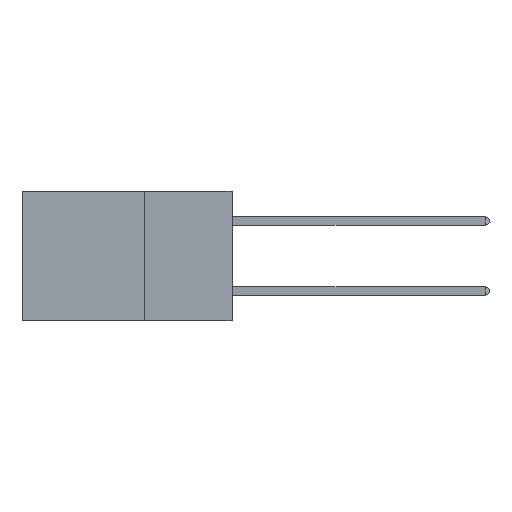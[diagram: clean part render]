
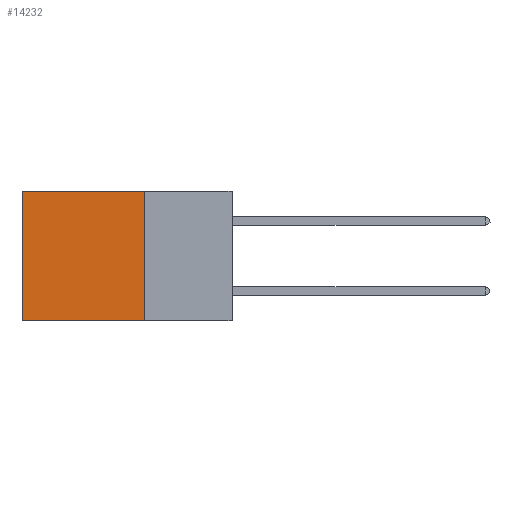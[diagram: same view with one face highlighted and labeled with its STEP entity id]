
A CAD part, left-side view. The second image highlights one B-rep face of the part: STEP entity #14232.
In plain terms, the highlighted planar face has unit normal (-1, 0, 0).
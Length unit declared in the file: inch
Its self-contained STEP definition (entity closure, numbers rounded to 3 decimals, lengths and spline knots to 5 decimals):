
#116 = DIRECTION ( 'NONE',  ( 0., 1., 0. ) ) ;
#477 = VERTEX_POINT ( 'NONE', #4011 ) ;
#758 = CARTESIAN_POINT ( 'NONE',  ( 0.2875, 0.25, 0. ) ) ;
#1013 = CARTESIAN_POINT ( 'NONE',  ( 0.2875, 0.25, -0.37 ) ) ;
#1071 = VERTEX_POINT ( 'NONE', #6090 ) ;
#1151 = ORIENTED_EDGE ( 'NONE', *, *, #7719, .T. ) ;
#1705 = ORIENTED_EDGE ( 'NONE', *, *, #3488, .T. ) ;
#3488 = EDGE_CURVE ( 'NONE', #13494, #477, #8154, .T. ) ;
#3638 = DIRECTION ( 'NONE',  ( 0., 0., -1. ) ) ;
#4011 = CARTESIAN_POINT ( 'NONE',  ( 0.2875, 0.6, 0. ) ) ;
#4682 = DIRECTION ( 'NONE',  ( 0., 1., 0. ) ) ;
#4878 = ORIENTED_EDGE ( 'NONE', *, *, #13527, .F. ) ;
#6062 = LINE ( 'NONE', #10101, #14825 ) ;
#6090 = CARTESIAN_POINT ( 'NONE',  ( 0.2875, 0.6, -0.37 ) ) ;
#6295 = LINE ( 'NONE', #1013, #7055 ) ;
#7055 = VECTOR ( 'NONE', #4682, 39.37008 ) ;
#7719 = EDGE_CURVE ( 'NONE', #477, #1071, #14773, .T. ) ;
#8154 = LINE ( 'NONE', #13543, #9310 ) ;
#8267 = VECTOR ( 'NONE', #8387, 39.37008 ) ;
#8387 = DIRECTION ( 'NONE',  ( 0., 0., -1. ) ) ;
#9310 = VECTOR ( 'NONE', #116, 39.37008 ) ;
#9897 = FACE_OUTER_BOUND ( 'NONE', #14467, .T. ) ;
#10101 = CARTESIAN_POINT ( 'NONE',  ( 0.2875, 0.25, 0. ) ) ;
#10247 = CARTESIAN_POINT ( 'NONE',  ( 0.2875, 0.25, -0.37 ) ) ;
#10675 = PLANE ( 'NONE',  #13339 ) ;
#10773 = CARTESIAN_POINT ( 'NONE',  ( 0.2875, 0.25, 0. ) ) ;
#10826 = ORIENTED_EDGE ( 'NONE', *, *, #12440, .F. ) ;
#11347 = DIRECTION ( 'NONE',  ( 0., 0., -1. ) ) ;
#12440 = EDGE_CURVE ( 'NONE', #13494, #14546, #6062, .T. ) ;
#13339 = AXIS2_PLACEMENT_3D ( 'NONE', #10773, #14583, #3638 ) ;
#13494 = VERTEX_POINT ( 'NONE', #758 ) ;
#13527 = EDGE_CURVE ( 'NONE', #14546, #1071, #6295, .T. ) ;
#13543 = CARTESIAN_POINT ( 'NONE',  ( 0.2875, 0.25, 0. ) ) ;
#14232 = ADVANCED_FACE ( 'NONE', ( #9897 ), #10675, .F. ) ;
#14386 = CARTESIAN_POINT ( 'NONE',  ( 0.2875, 0.6, 0. ) ) ;
#14467 = EDGE_LOOP ( 'NONE', ( #1151, #4878, #10826, #1705 ) ) ;
#14546 = VERTEX_POINT ( 'NONE', #10247 ) ;
#14583 = DIRECTION ( 'NONE',  ( 1., 0., 0. ) ) ;
#14773 = LINE ( 'NONE', #14386, #8267 ) ;
#14825 = VECTOR ( 'NONE', #11347, 39.37008 ) ;
